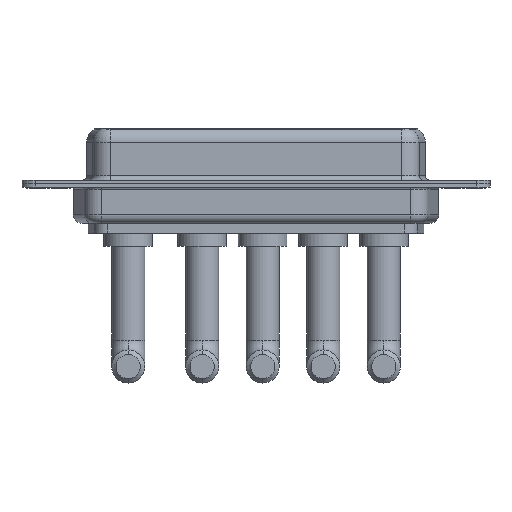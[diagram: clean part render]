
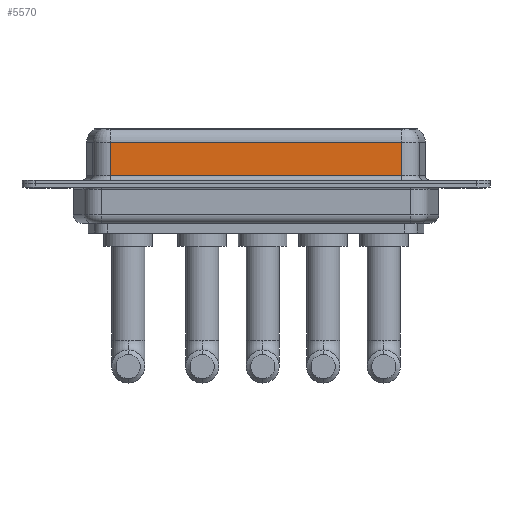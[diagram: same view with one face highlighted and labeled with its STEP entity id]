
A CAD part, front view. The second image highlights one B-rep face of the part: STEP entity #5570.
In plain terms, the highlighted planar face has unit normal (0, -1, 0).
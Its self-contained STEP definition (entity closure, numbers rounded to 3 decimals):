
#109 = DIRECTION ( 'NONE',  ( 0., 0., 1. ) ) ;
#250 = VECTOR ( 'NONE', #3815, 1000. ) ;
#603 = LINE ( 'NONE', #2999, #2585 ) ;
#1017 = CARTESIAN_POINT ( 'NONE',  ( 40.037, -3.95, 4.65 ) ) ;
#1146 = LINE ( 'NONE', #5289, #2503 ) ;
#1626 = DIRECTION ( 'NONE',  ( 0., 1., 0. ) ) ;
#2147 = LINE ( 'NONE', #9843, #250 ) ;
#2503 = VECTOR ( 'NONE', #9609, 1000. ) ;
#2585 = VECTOR ( 'NONE', #5545, 1000. ) ;
#2710 = ORIENTED_EDGE ( 'NONE', *, *, #8916, .T. ) ;
#2719 = EDGE_CURVE ( 'NONE', #2997, #8052, #5375, .T. ) ;
#2997 = VERTEX_POINT ( 'NONE', #1017 ) ;
#2999 = CARTESIAN_POINT ( 'NONE',  ( 40.037, -3.95, 0.9 ) ) ;
#3062 = CARTESIAN_POINT ( 'NONE',  ( 7.013, -3.95, 4.65 ) ) ;
#3464 = VERTEX_POINT ( 'NONE', #10298 ) ;
#3815 = DIRECTION ( 'NONE',  ( 0., 0., -1. ) ) ;
#3986 = CARTESIAN_POINT ( 'NONE',  ( 7.013, -3.95, 0.9 ) ) ;
#4554 = DIRECTION ( 'NONE',  ( -1., 0., 0. ) ) ;
#4570 = VERTEX_POINT ( 'NONE', #3986 ) ;
#5289 = CARTESIAN_POINT ( 'NONE',  ( 40.037, -3.95, 6.4 ) ) ;
#5375 = LINE ( 'NONE', #7033, #10124 ) ;
#5470 = EDGE_CURVE ( 'NONE', #4570, #3464, #603, .T. ) ;
#5545 = DIRECTION ( 'NONE',  ( 1., 0., 0. ) ) ;
#5570 = ADVANCED_FACE ( 'NONE', ( #10897 ), #9325, .F. ) ;
#6330 = EDGE_LOOP ( 'NONE', ( #8751, #9488, #2710, #10645 ) ) ;
#6662 = CARTESIAN_POINT ( 'NONE',  ( 40.037, -3.95, 6.4 ) ) ;
#7033 = CARTESIAN_POINT ( 'NONE',  ( 40.037, -3.95, 4.65 ) ) ;
#8052 = VERTEX_POINT ( 'NONE', #3062 ) ;
#8751 = ORIENTED_EDGE ( 'NONE', *, *, #9323, .F. ) ;
#8916 = EDGE_CURVE ( 'NONE', #8052, #4570, #2147, .T. ) ;
#9323 = EDGE_CURVE ( 'NONE', #2997, #3464, #1146, .T. ) ;
#9325 = PLANE ( 'NONE',  #9651 ) ;
#9488 = ORIENTED_EDGE ( 'NONE', *, *, #2719, .T. ) ;
#9609 = DIRECTION ( 'NONE',  ( 0., 0., -1. ) ) ;
#9651 = AXIS2_PLACEMENT_3D ( 'NONE', #6662, #1626, #109 ) ;
#9843 = CARTESIAN_POINT ( 'NONE',  ( 7.013, -3.95, 6.4 ) ) ;
#10124 = VECTOR ( 'NONE', #4554, 1000. ) ;
#10298 = CARTESIAN_POINT ( 'NONE',  ( 40.037, -3.95, 0.9 ) ) ;
#10645 = ORIENTED_EDGE ( 'NONE', *, *, #5470, .T. ) ;
#10897 = FACE_OUTER_BOUND ( 'NONE', #6330, .T. ) ;
